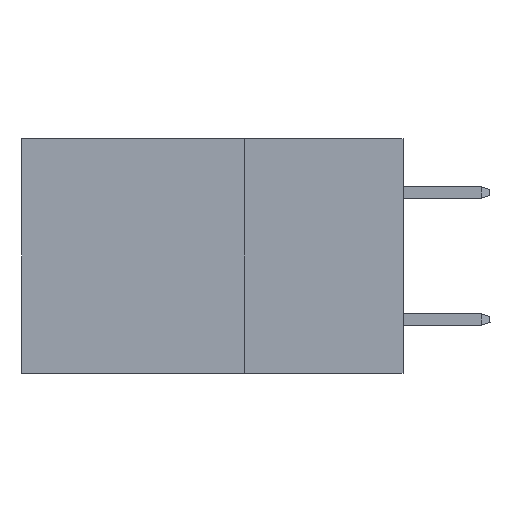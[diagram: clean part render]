
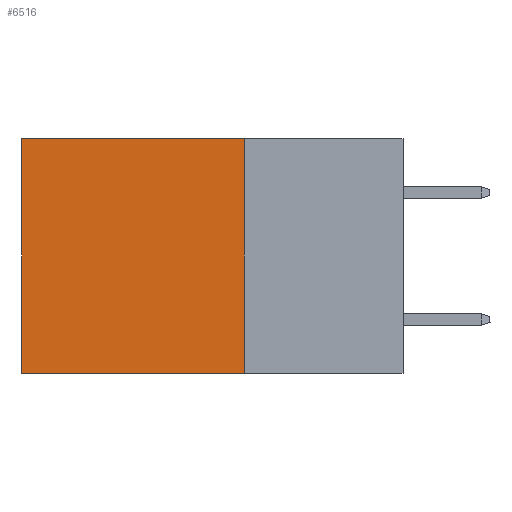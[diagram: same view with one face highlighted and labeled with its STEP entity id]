
A CAD part, left-side view. The second image highlights one B-rep face of the part: STEP entity #6516.
In plain terms, the highlighted planar face has unit normal (-1, 0, 0).
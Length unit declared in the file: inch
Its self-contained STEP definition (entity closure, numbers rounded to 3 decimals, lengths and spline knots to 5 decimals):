
#479 = CARTESIAN_POINT ( 'NONE',  ( 0.2875, 0.25, 0. ) ) ;
#618 = VECTOR ( 'NONE', #9864, 39.37008 ) ;
#642 = ORIENTED_EDGE ( 'NONE', *, *, #9288, .F. ) ;
#988 = VECTOR ( 'NONE', #9049, 39.37008 ) ;
#1208 = CARTESIAN_POINT ( 'NONE',  ( 0.2875, 0.25, -0.37 ) ) ;
#1748 = DIRECTION ( 'NONE',  ( 0., 0., -1. ) ) ;
#1860 = VERTEX_POINT ( 'NONE', #9629 ) ;
#1961 = LINE ( 'NONE', #12663, #13744 ) ;
#2626 = LINE ( 'NONE', #12592, #988 ) ;
#3062 = EDGE_LOOP ( 'NONE', ( #10342, #642, #13132, #3841 ) ) ;
#3712 = PLANE ( 'NONE',  #4005 ) ;
#3841 = ORIENTED_EDGE ( 'NONE', *, *, #6038, .T. ) ;
#4005 = AXIS2_PLACEMENT_3D ( 'NONE', #479, #4855, #13072 ) ;
#4148 = VERTEX_POINT ( 'NONE', #5876 ) ;
#4855 = DIRECTION ( 'NONE',  ( 1., 0., 0. ) ) ;
#5200 = EDGE_CURVE ( 'NONE', #1860, #4148, #1961, .T. ) ;
#5876 = CARTESIAN_POINT ( 'NONE',  ( 0.2875, 0.6, -0.37 ) ) ;
#5907 = FACE_OUTER_BOUND ( 'NONE', #3062, .T. ) ;
#6038 = EDGE_CURVE ( 'NONE', #8050, #1860, #2626, .T. ) ;
#6305 = VERTEX_POINT ( 'NONE', #8557 ) ;
#6516 = ADVANCED_FACE ( 'NONE', ( #5907 ), #3712, .F. ) ;
#6661 = VECTOR ( 'NONE', #7669, 39.37008 ) ;
#7669 = DIRECTION ( 'NONE',  ( 0., 1., 0. ) ) ;
#7808 = LINE ( 'NONE', #11098, #618 ) ;
#8050 = VERTEX_POINT ( 'NONE', #13715 ) ;
#8557 = CARTESIAN_POINT ( 'NONE',  ( 0.2875, 0.25, -0.37 ) ) ;
#9049 = DIRECTION ( 'NONE',  ( 0., 1., 0. ) ) ;
#9288 = EDGE_CURVE ( 'NONE', #6305, #4148, #13138, .T. ) ;
#9629 = CARTESIAN_POINT ( 'NONE',  ( 0.2875, 0.6, 0. ) ) ;
#9864 = DIRECTION ( 'NONE',  ( 0., 0., -1. ) ) ;
#10342 = ORIENTED_EDGE ( 'NONE', *, *, #5200, .T. ) ;
#11098 = CARTESIAN_POINT ( 'NONE',  ( 0.2875, 0.25, 0. ) ) ;
#11654 = EDGE_CURVE ( 'NONE', #8050, #6305, #7808, .T. ) ;
#12592 = CARTESIAN_POINT ( 'NONE',  ( 0.2875, 0.25, 0. ) ) ;
#12663 = CARTESIAN_POINT ( 'NONE',  ( 0.2875, 0.6, 0. ) ) ;
#13072 = DIRECTION ( 'NONE',  ( 0., 0., -1. ) ) ;
#13132 = ORIENTED_EDGE ( 'NONE', *, *, #11654, .F. ) ;
#13138 = LINE ( 'NONE', #1208, #6661 ) ;
#13715 = CARTESIAN_POINT ( 'NONE',  ( 0.2875, 0.25, 0. ) ) ;
#13744 = VECTOR ( 'NONE', #1748, 39.37008 ) ;
